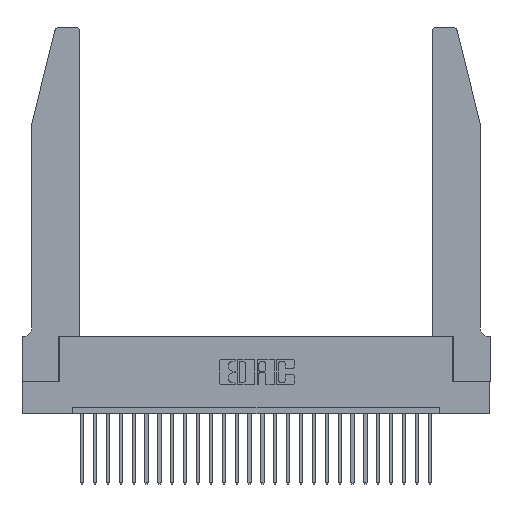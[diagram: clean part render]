
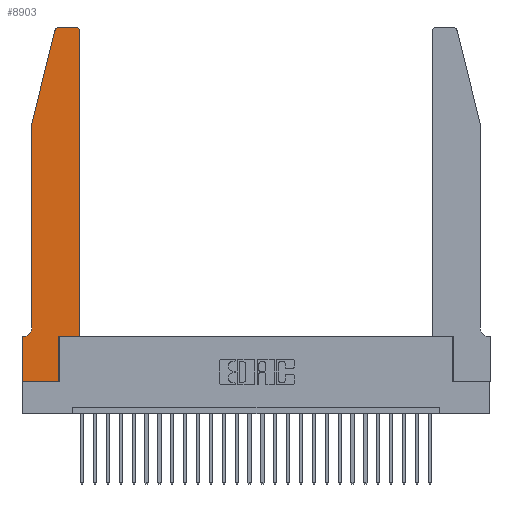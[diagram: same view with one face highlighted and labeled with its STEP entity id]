
A CAD part, top view. The second image highlights one B-rep face of the part: STEP entity #8903.
In plain terms, the highlighted planar face has unit normal (0, 0, 1).
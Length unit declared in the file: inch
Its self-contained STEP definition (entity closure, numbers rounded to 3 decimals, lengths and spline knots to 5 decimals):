
#345 = CARTESIAN_POINT ( 'NONE',  ( 0.2865, 0., 0.37 ) ) ;
#586 = EDGE_CURVE ( 'NONE', #11818, #5386, #2369, .T. ) ;
#611 = ORIENTED_EDGE ( 'NONE', *, *, #12445, .T. ) ;
#708 = CARTESIAN_POINT ( 'NONE',  ( 0.0755, 2., 0.37 ) ) ;
#908 = DIRECTION ( 'NONE',  ( 0., 1., 0. ) ) ;
#1478 = ORIENTED_EDGE ( 'NONE', *, *, #11481, .T. ) ;
#1835 = CARTESIAN_POINT ( 'NONE',  ( 0.0755, 0.42, 0.37 ) ) ;
#2119 = CARTESIAN_POINT ( 'NONE',  ( 0., 0., 0.37 ) ) ;
#2130 = DIRECTION ( 'NONE',  ( 0., 0., -1. ) ) ;
#2369 = LINE ( 'NONE', #2119, #5699 ) ;
#2885 = EDGE_CURVE ( 'NONE', #6565, #11818, #15627, .T. ) ;
#3068 = DIRECTION ( 'NONE',  ( 1., 0., 0. ) ) ;
#3330 = FACE_OUTER_BOUND ( 'NONE', #12100, .T. ) ;
#4263 = AXIS2_PLACEMENT_3D ( 'NONE', #20151, #26716, #18276 ) ;
#4677 = CARTESIAN_POINT ( 'NONE',  ( 0., 0.35, 0.37 ) ) ;
#4754 = ORIENTED_EDGE ( 'NONE', *, *, #20756, .T. ) ;
#4843 = CARTESIAN_POINT ( 'NONE',  ( 0.4505, 0.35, 0.37 ) ) ;
#5216 = ORIENTED_EDGE ( 'NONE', *, *, #14178, .T. ) ;
#5232 = VECTOR ( 'NONE', #26874, 39.37008 ) ;
#5386 = VERTEX_POINT ( 'NONE', #16609 ) ;
#5699 = VECTOR ( 'NONE', #23988, 39.37008 ) ;
#5739 = EDGE_CURVE ( 'NONE', #8179, #6565, #15590, .T. ) ;
#6565 = VERTEX_POINT ( 'NONE', #20290 ) ;
#6825 = VECTOR ( 'NONE', #7207, 39.37008 ) ;
#7207 = DIRECTION ( 'NONE',  ( -0.239, -0.971, 0. ) ) ;
#7212 = AXIS2_PLACEMENT_3D ( 'NONE', #10571, #2130, #18732 ) ;
#7381 = DIRECTION ( 'NONE',  ( -1., 0., 0. ) ) ;
#7543 = LINE ( 'NONE', #15731, #24286 ) ;
#8179 = VERTEX_POINT ( 'NONE', #1835 ) ;
#8452 = CARTESIAN_POINT ( 'NONE',  ( 0.0755, 2., 0.37 ) ) ;
#8455 = VERTEX_POINT ( 'NONE', #10967 ) ;
#8664 = AXIS2_PLACEMENT_3D ( 'NONE', #16853, #18986, #20971 ) ;
#8903 = ADVANCED_FACE ( 'NONE', ( #3330 ), #24343, .T. ) ;
#9019 = ORIENTED_EDGE ( 'NONE', *, *, #26529, .T. ) ;
#9250 = DIRECTION ( 'NONE',  ( 1., 0., 0. ) ) ;
#9381 = CARTESIAN_POINT ( 'NONE',  ( 0., 0.35, 0.37 ) ) ;
#9611 = CIRCLE ( 'NONE', #4263, 0.03 ) ;
#10461 = ORIENTED_EDGE ( 'NONE', *, *, #5739, .T. ) ;
#10571 = CARTESIAN_POINT ( 'NONE',  ( 0.0055, 0.42, 0.37 ) ) ;
#10967 = CARTESIAN_POINT ( 'NONE',  ( 0.25487, 2.72718, 0.37 ) ) ;
#11098 = LINE ( 'NONE', #4843, #16735 ) ;
#11481 = EDGE_CURVE ( 'NONE', #16781, #8455, #9611, .T. ) ;
#11545 = DIRECTION ( 'NONE',  ( 0., 0., 1. ) ) ;
#11818 = VERTEX_POINT ( 'NONE', #4677 ) ;
#11999 = VERTEX_POINT ( 'NONE', #23445 ) ;
#12100 = EDGE_LOOP ( 'NONE', ( #611, #1478, #5216, #12973, #10461, #21006, #17547, #25178, #9019, #24581, #18980, #4754 ) ) ;
#12242 = VERTEX_POINT ( 'NONE', #14391 ) ;
#12445 = EDGE_CURVE ( 'NONE', #11999, #16781, #20252, .T. ) ;
#12973 = ORIENTED_EDGE ( 'NONE', *, *, #24807, .T. ) ;
#13172 = EDGE_CURVE ( 'NONE', #16704, #12242, #7543, .T. ) ;
#13177 = LINE ( 'NONE', #708, #6825 ) ;
#14178 = EDGE_CURVE ( 'NONE', #8455, #26373, #13177, .T. ) ;
#14391 = CARTESIAN_POINT ( 'NONE',  ( 0.4505, 2.72, 0.37 ) ) ;
#15325 = CARTESIAN_POINT ( 'NONE',  ( 0.284, 2.75, 0.37 ) ) ;
#15494 = EDGE_CURVE ( 'NONE', #27197, #16704, #11098, .T. ) ;
#15590 = CIRCLE ( 'NONE', #7212, 0.07 ) ;
#15627 = LINE ( 'NONE', #18162, #5232 ) ;
#15731 = CARTESIAN_POINT ( 'NONE',  ( 0.4505, 0.35, 0.37 ) ) ;
#15989 = CARTESIAN_POINT ( 'NONE',  ( 0.0755, 2., 0.37 ) ) ;
#16269 = CARTESIAN_POINT ( 'NONE',  ( 0.2605, 2.75, 0.37 ) ) ;
#16609 = CARTESIAN_POINT ( 'NONE',  ( 0., 0., 0.37 ) ) ;
#16704 = VERTEX_POINT ( 'NONE', #18879 ) ;
#16735 = VECTOR ( 'NONE', #3068, 39.37008 ) ;
#16781 = VERTEX_POINT ( 'NONE', #15325 ) ;
#16853 = CARTESIAN_POINT ( 'NONE',  ( 0.4205, 2.72, 0.37 ) ) ;
#17547 = ORIENTED_EDGE ( 'NONE', *, *, #586, .T. ) ;
#17853 = LINE ( 'NONE', #19597, #21538 ) ;
#18162 = CARTESIAN_POINT ( 'NONE',  ( 0.0755, 0.35, 0.37 ) ) ;
#18276 = DIRECTION ( 'NONE',  ( 1., 0., 0. ) ) ;
#18627 = VERTEX_POINT ( 'NONE', #345 ) ;
#18732 = DIRECTION ( 'NONE',  ( -1., 0., 0. ) ) ;
#18763 = CIRCLE ( 'NONE', #8664, 0.03 ) ;
#18879 = CARTESIAN_POINT ( 'NONE',  ( 0.4505, 0.35, 0.37 ) ) ;
#18980 = ORIENTED_EDGE ( 'NONE', *, *, #13172, .T. ) ;
#18986 = DIRECTION ( 'NONE',  ( 0., 0., 1. ) ) ;
#19597 = CARTESIAN_POINT ( 'NONE',  ( 0., 0., 0.37 ) ) ;
#19619 = DIRECTION ( 'NONE',  ( 0., 1., 0. ) ) ;
#19876 = CARTESIAN_POINT ( 'NONE',  ( 0.2865, 0.35, 0.37 ) ) ;
#20151 = CARTESIAN_POINT ( 'NONE',  ( 0.284, 2.72, 0.37 ) ) ;
#20208 = LINE ( 'NONE', #15989, #25917 ) ;
#20252 = LINE ( 'NONE', #16269, #22951 ) ;
#20264 = DIRECTION ( 'NONE',  ( 0., -1., 0. ) ) ;
#20290 = CARTESIAN_POINT ( 'NONE',  ( 0.0055, 0.35, 0.37 ) ) ;
#20756 = EDGE_CURVE ( 'NONE', #12242, #11999, #18763, .T. ) ;
#20971 = DIRECTION ( 'NONE',  ( 1., 0., 0. ) ) ;
#21006 = ORIENTED_EDGE ( 'NONE', *, *, #2885, .T. ) ;
#21538 = VECTOR ( 'NONE', #9250, 39.37008 ) ;
#21902 = DIRECTION ( 'NONE',  ( 1., 0., 0. ) ) ;
#22951 = VECTOR ( 'NONE', #7381, 39.37008 ) ;
#23445 = CARTESIAN_POINT ( 'NONE',  ( 0.4205, 2.75, 0.37 ) ) ;
#23988 = DIRECTION ( 'NONE',  ( 0., -1., 0. ) ) ;
#24286 = VECTOR ( 'NONE', #908, 39.37008 ) ;
#24343 = PLANE ( 'NONE',  #27316 ) ;
#24581 = ORIENTED_EDGE ( 'NONE', *, *, #15494, .T. ) ;
#24807 = EDGE_CURVE ( 'NONE', #26373, #8179, #20208, .T. ) ;
#24833 = VECTOR ( 'NONE', #19619, 39.37008 ) ;
#25178 = ORIENTED_EDGE ( 'NONE', *, *, #25203, .T. ) ;
#25203 = EDGE_CURVE ( 'NONE', #5386, #18627, #17853, .T. ) ;
#25499 = LINE ( 'NONE', #26094, #24833 ) ;
#25917 = VECTOR ( 'NONE', #20264, 39.37008 ) ;
#26094 = CARTESIAN_POINT ( 'NONE',  ( 0.2865, 0.35, 0.37 ) ) ;
#26373 = VERTEX_POINT ( 'NONE', #8452 ) ;
#26529 = EDGE_CURVE ( 'NONE', #18627, #27197, #25499, .T. ) ;
#26716 = DIRECTION ( 'NONE',  ( 0., 0., 1. ) ) ;
#26874 = DIRECTION ( 'NONE',  ( -1., 0., 0. ) ) ;
#27197 = VERTEX_POINT ( 'NONE', #19876 ) ;
#27316 = AXIS2_PLACEMENT_3D ( 'NONE', #9381, #11545, #21902 ) ;
